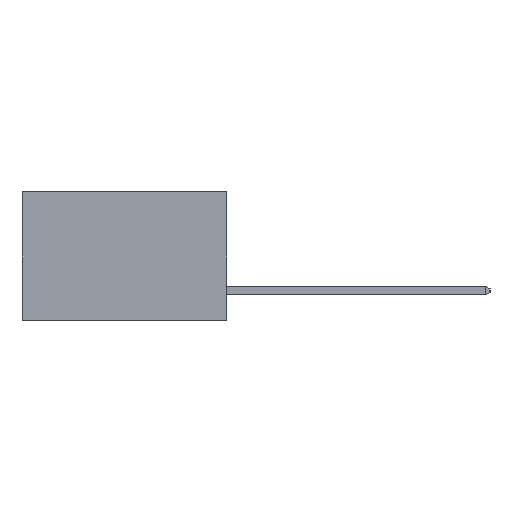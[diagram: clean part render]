
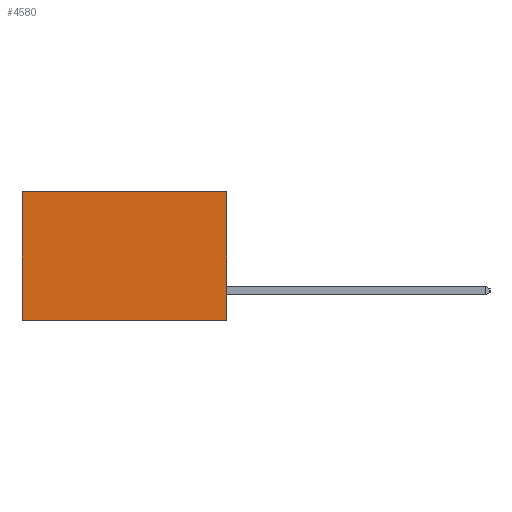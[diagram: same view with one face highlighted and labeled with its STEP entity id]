
A CAD part, left-side view. The second image highlights one B-rep face of the part: STEP entity #4580.
In plain terms, the highlighted planar face has unit normal (-1, 0, 0).
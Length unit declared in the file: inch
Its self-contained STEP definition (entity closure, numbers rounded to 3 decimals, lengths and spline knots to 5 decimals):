
#1003 = EDGE_CURVE ( 'NONE', #4821, #21082, #11762, .T. ) ;
#1435 = ORIENTED_EDGE ( 'NONE', *, *, #1003, .F. ) ;
#2243 = DIRECTION ( 'NONE',  ( 0., 0., -1. ) ) ;
#2291 = DIRECTION ( 'NONE',  ( 1., 0., 0. ) ) ;
#2929 = PLANE ( 'NONE',  #31904 ) ;
#3263 = CARTESIAN_POINT ( 'NONE',  ( 0.277, 0., -0.37 ) ) ;
#3267 = CARTESIAN_POINT ( 'NONE',  ( 0.277, 0., -0.37 ) ) ;
#3376 = DIRECTION ( 'NONE',  ( 0., 0., -1. ) ) ;
#4115 = ORIENTED_EDGE ( 'NONE', *, *, #26591, .T. ) ;
#4580 = ADVANCED_FACE ( 'NONE', ( #26801 ), #2929, .F. ) ;
#4609 = EDGE_LOOP ( 'NONE', ( #4115, #1435, #17504, #20588 ) ) ;
#4821 = VERTEX_POINT ( 'NONE', #7191 ) ;
#5221 = VECTOR ( 'NONE', #15063, 39.37008 ) ;
#5790 = CARTESIAN_POINT ( 'NONE',  ( 0.277, 0., 0. ) ) ;
#6412 = CARTESIAN_POINT ( 'NONE',  ( 0.277, 0.59, -0.37 ) ) ;
#7191 = CARTESIAN_POINT ( 'NONE',  ( 0.277, 0., -0.37 ) ) ;
#7589 = EDGE_CURVE ( 'NONE', #30924, #4821, #11418, .T. ) ;
#10960 = VECTOR ( 'NONE', #24255, 39.37008 ) ;
#11418 = LINE ( 'NONE', #3263, #24339 ) ;
#11762 = LINE ( 'NONE', #18366, #10960 ) ;
#12074 = LINE ( 'NONE', #12457, #5221 ) ;
#12457 = CARTESIAN_POINT ( 'NONE',  ( 0.277, 0., 0. ) ) ;
#12778 = CARTESIAN_POINT ( 'NONE',  ( 0.277, 0.59, 0. ) ) ;
#13267 = EDGE_CURVE ( 'NONE', #30924, #13374, #12074, .T. ) ;
#13374 = VERTEX_POINT ( 'NONE', #12778 ) ;
#15063 = DIRECTION ( 'NONE',  ( 0., 1., 0. ) ) ;
#16245 = LINE ( 'NONE', #17432, #28985 ) ;
#17432 = CARTESIAN_POINT ( 'NONE',  ( 0.277, 0.59, -0.37 ) ) ;
#17504 = ORIENTED_EDGE ( 'NONE', *, *, #7589, .F. ) ;
#18366 = CARTESIAN_POINT ( 'NONE',  ( 0.277, 0., -0.37 ) ) ;
#20038 = DIRECTION ( 'NONE',  ( 0., 0., -1. ) ) ;
#20588 = ORIENTED_EDGE ( 'NONE', *, *, #13267, .T. ) ;
#21082 = VERTEX_POINT ( 'NONE', #6412 ) ;
#24255 = DIRECTION ( 'NONE',  ( 0., 1., 0. ) ) ;
#24339 = VECTOR ( 'NONE', #3376, 39.37008 ) ;
#26591 = EDGE_CURVE ( 'NONE', #13374, #21082, #16245, .T. ) ;
#26801 = FACE_OUTER_BOUND ( 'NONE', #4609, .T. ) ;
#28985 = VECTOR ( 'NONE', #20038, 39.37008 ) ;
#30924 = VERTEX_POINT ( 'NONE', #5790 ) ;
#31904 = AXIS2_PLACEMENT_3D ( 'NONE', #3267, #2291, #2243 ) ;
